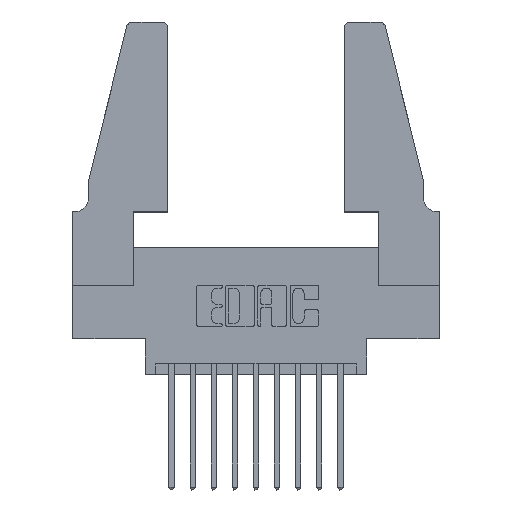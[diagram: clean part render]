
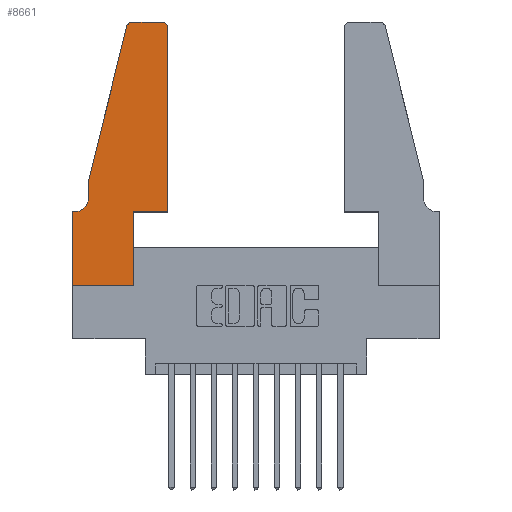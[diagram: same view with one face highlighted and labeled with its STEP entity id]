
A CAD part, top view. The second image highlights one B-rep face of the part: STEP entity #8661.
In plain terms, the highlighted planar face has unit normal (0, 0, 1).
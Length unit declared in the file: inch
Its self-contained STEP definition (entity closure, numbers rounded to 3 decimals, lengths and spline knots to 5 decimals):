
#24 = CARTESIAN_POINT ( 'NONE',  ( 0.284, 1.25, 0.37 ) ) ;
#96 = CARTESIAN_POINT ( 'NONE',  ( 0.4505, 0.35, 0.37 ) ) ;
#128 = DIRECTION ( 'NONE',  ( 0., -1., 0. ) ) ;
#137 = VERTEX_POINT ( 'NONE', #9376 ) ;
#185 = CARTESIAN_POINT ( 'NONE',  ( 0.2865, 0.35, 0.37 ) ) ;
#256 = CARTESIAN_POINT ( 'NONE',  ( 0.4505, 0.35, 0.37 ) ) ;
#344 = EDGE_CURVE ( 'NONE', #2412, #11639, #13516, .T. ) ;
#498 = CARTESIAN_POINT ( 'NONE',  ( 0.0755, 0.42, 0.37 ) ) ;
#579 = ORIENTED_EDGE ( 'NONE', *, *, #12379, .T. ) ;
#656 = AXIS2_PLACEMENT_3D ( 'NONE', #7963, #12219, #6876 ) ;
#713 = ORIENTED_EDGE ( 'NONE', *, *, #8536, .T. ) ;
#887 = CARTESIAN_POINT ( 'NONE',  ( 0.0755, 0.35, 0.37 ) ) ;
#1089 = ORIENTED_EDGE ( 'NONE', *, *, #2158, .T. ) ;
#1293 = PLANE ( 'NONE',  #5789 ) ;
#1519 = VERTEX_POINT ( 'NONE', #256 ) ;
#1520 = DIRECTION ( 'NONE',  ( 1., 0., 0. ) ) ;
#1667 = CARTESIAN_POINT ( 'NONE',  ( 0.25487, 1.22718, 0.37 ) ) ;
#2043 = VERTEX_POINT ( 'NONE', #10793 ) ;
#2094 = LINE ( 'NONE', #7899, #13143 ) ;
#2133 = ORIENTED_EDGE ( 'NONE', *, *, #344, .T. ) ;
#2158 = EDGE_CURVE ( 'NONE', #1519, #12742, #2094, .T. ) ;
#2412 = VERTEX_POINT ( 'NONE', #24 ) ;
#2608 = CIRCLE ( 'NONE', #5452, 0.03 ) ;
#2717 = EDGE_CURVE ( 'NONE', #9230, #2043, #6122, .T. ) ;
#3054 = LINE ( 'NONE', #13271, #10102 ) ;
#3170 = LINE ( 'NONE', #11519, #8540 ) ;
#3433 = CARTESIAN_POINT ( 'NONE',  ( 0., 0.35, 0.37 ) ) ;
#3694 = VERTEX_POINT ( 'NONE', #13079 ) ;
#3807 = CARTESIAN_POINT ( 'NONE',  ( 0., 0., 0.37 ) ) ;
#4015 = DIRECTION ( 'NONE',  ( 0., 0., 1. ) ) ;
#4039 = VECTOR ( 'NONE', #12586, 39.37008 ) ;
#4126 = LINE ( 'NONE', #8763, #7300 ) ;
#4345 = ORIENTED_EDGE ( 'NONE', *, *, #10127, .T. ) ;
#4628 = CIRCLE ( 'NONE', #656, 0.07 ) ;
#4776 = EDGE_CURVE ( 'NONE', #2043, #137, #11454, .T. ) ;
#5104 = ORIENTED_EDGE ( 'NONE', *, *, #2717, .T. ) ;
#5174 = ORIENTED_EDGE ( 'NONE', *, *, #6826, .T. ) ;
#5250 = LINE ( 'NONE', #96, #9419 ) ;
#5326 = CARTESIAN_POINT ( 'NONE',  ( 0.4505, 1.22, 0.37 ) ) ;
#5353 = EDGE_LOOP ( 'NONE', ( #11053, #2133, #9680, #4345, #713, #5104, #7265, #8318, #5174, #579, #1089, #5525 ) ) ;
#5387 = DIRECTION ( 'NONE',  ( 0., 0., 1. ) ) ;
#5452 = AXIS2_PLACEMENT_3D ( 'NONE', #7712, #5696, #13150 ) ;
#5525 = ORIENTED_EDGE ( 'NONE', *, *, #8786, .T. ) ;
#5696 = DIRECTION ( 'NONE',  ( 0., 0., 1. ) ) ;
#5789 = AXIS2_PLACEMENT_3D ( 'NONE', #3433, #5387, #1520 ) ;
#6044 = DIRECTION ( 'NONE',  ( 0., -1., 0. ) ) ;
#6122 = LINE ( 'NONE', #887, #12638 ) ;
#6631 = CARTESIAN_POINT ( 'NONE',  ( 0.2865, 0., 0.37 ) ) ;
#6657 = EDGE_CURVE ( 'NONE', #7135, #2412, #7547, .T. ) ;
#6705 = CARTESIAN_POINT ( 'NONE',  ( 0.0055, 0.35, 0.37 ) ) ;
#6794 = DIRECTION ( 'NONE',  ( 1., 0., 0. ) ) ;
#6826 = EDGE_CURVE ( 'NONE', #9888, #12427, #3170, .T. ) ;
#6876 = DIRECTION ( 'NONE',  ( -1., 0., 0. ) ) ;
#7135 = VERTEX_POINT ( 'NONE', #9876 ) ;
#7208 = AXIS2_PLACEMENT_3D ( 'NONE', #10394, #4015, #11512 ) ;
#7236 = DIRECTION ( 'NONE',  ( 0., 1., 0. ) ) ;
#7265 = ORIENTED_EDGE ( 'NONE', *, *, #4776, .T. ) ;
#7300 = VECTOR ( 'NONE', #128, 39.37008 ) ;
#7547 = LINE ( 'NONE', #11886, #13055 ) ;
#7712 = CARTESIAN_POINT ( 'NONE',  ( 0.4205, 1.22, 0.37 ) ) ;
#7899 = CARTESIAN_POINT ( 'NONE',  ( 0.4505, 0.35, 0.37 ) ) ;
#7947 = VECTOR ( 'NONE', #6044, 39.37008 ) ;
#7963 = CARTESIAN_POINT ( 'NONE',  ( 0.0055, 0.42, 0.37 ) ) ;
#8299 = DIRECTION ( 'NONE',  ( -1., 0., 0. ) ) ;
#8318 = ORIENTED_EDGE ( 'NONE', *, *, #11579, .T. ) ;
#8536 = EDGE_CURVE ( 'NONE', #11192, #9230, #4628, .T. ) ;
#8540 = VECTOR ( 'NONE', #7236, 39.37008 ) ;
#8661 = ADVANCED_FACE ( 'NONE', ( #10140 ), #1293, .T. ) ;
#8763 = CARTESIAN_POINT ( 'NONE',  ( 0.0755, 0.5, 0.37 ) ) ;
#8786 = EDGE_CURVE ( 'NONE', #12742, #7135, #2608, .T. ) ;
#8961 = DIRECTION ( 'NONE',  ( 0., 1., 0. ) ) ;
#9230 = VERTEX_POINT ( 'NONE', #6705 ) ;
#9376 = CARTESIAN_POINT ( 'NONE',  ( 0., 0., 0.37 ) ) ;
#9419 = VECTOR ( 'NONE', #12981, 39.37008 ) ;
#9502 = CARTESIAN_POINT ( 'NONE',  ( 0.0755, 0.5, 0.37 ) ) ;
#9680 = ORIENTED_EDGE ( 'NONE', *, *, #13617, .T. ) ;
#9876 = CARTESIAN_POINT ( 'NONE',  ( 0.4205, 1.25, 0.37 ) ) ;
#9888 = VERTEX_POINT ( 'NONE', #6631 ) ;
#10102 = VECTOR ( 'NONE', #6794, 39.37008 ) ;
#10127 = EDGE_CURVE ( 'NONE', #3694, #11192, #4126, .T. ) ;
#10140 = FACE_OUTER_BOUND ( 'NONE', #5353, .T. ) ;
#10377 = LINE ( 'NONE', #9502, #4039 ) ;
#10394 = CARTESIAN_POINT ( 'NONE',  ( 0.284, 1.22, 0.37 ) ) ;
#10793 = CARTESIAN_POINT ( 'NONE',  ( 0., 0.35, 0.37 ) ) ;
#11053 = ORIENTED_EDGE ( 'NONE', *, *, #6657, .T. ) ;
#11192 = VERTEX_POINT ( 'NONE', #498 ) ;
#11377 = DIRECTION ( 'NONE',  ( -1., 0., 0. ) ) ;
#11454 = LINE ( 'NONE', #3807, #7947 ) ;
#11512 = DIRECTION ( 'NONE',  ( 1., 0., 0. ) ) ;
#11519 = CARTESIAN_POINT ( 'NONE',  ( 0.2865, 0.35, 0.37 ) ) ;
#11579 = EDGE_CURVE ( 'NONE', #137, #9888, #3054, .T. ) ;
#11639 = VERTEX_POINT ( 'NONE', #1667 ) ;
#11886 = CARTESIAN_POINT ( 'NONE',  ( 0.2605, 1.25, 0.37 ) ) ;
#12219 = DIRECTION ( 'NONE',  ( 0., 0., -1. ) ) ;
#12379 = EDGE_CURVE ( 'NONE', #12427, #1519, #5250, .T. ) ;
#12427 = VERTEX_POINT ( 'NONE', #185 ) ;
#12586 = DIRECTION ( 'NONE',  ( -0.239, -0.971, 0. ) ) ;
#12638 = VECTOR ( 'NONE', #8299, 39.37008 ) ;
#12742 = VERTEX_POINT ( 'NONE', #5326 ) ;
#12981 = DIRECTION ( 'NONE',  ( 1., 0., 0. ) ) ;
#13055 = VECTOR ( 'NONE', #11377, 39.37008 ) ;
#13079 = CARTESIAN_POINT ( 'NONE',  ( 0.0755, 0.5, 0.37 ) ) ;
#13143 = VECTOR ( 'NONE', #8961, 39.37008 ) ;
#13150 = DIRECTION ( 'NONE',  ( 1., 0., 0. ) ) ;
#13271 = CARTESIAN_POINT ( 'NONE',  ( 0., 0., 0.37 ) ) ;
#13516 = CIRCLE ( 'NONE', #7208, 0.03 ) ;
#13617 = EDGE_CURVE ( 'NONE', #11639, #3694, #10377, .T. ) ;
